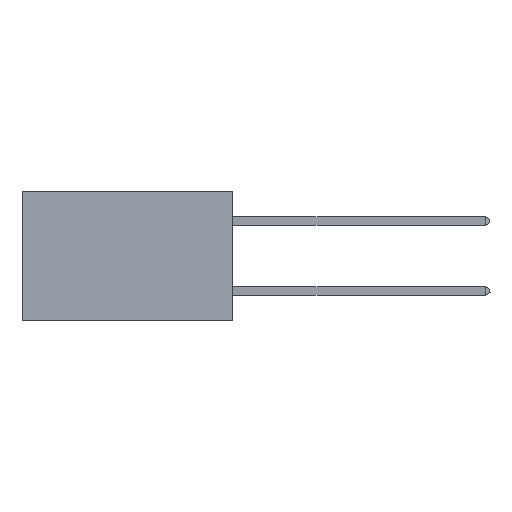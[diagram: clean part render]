
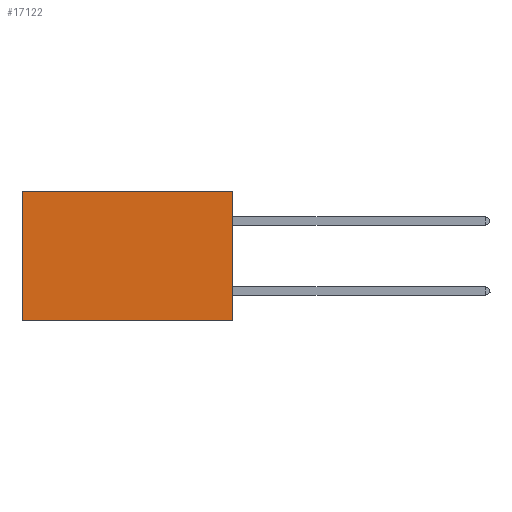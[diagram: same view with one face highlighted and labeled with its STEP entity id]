
A CAD part, left-side view. The second image highlights one B-rep face of the part: STEP entity #17122.
In plain terms, the highlighted planar face has unit normal (-1, 0, 0).
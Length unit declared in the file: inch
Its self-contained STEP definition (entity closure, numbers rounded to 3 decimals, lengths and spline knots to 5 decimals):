
#410 = CARTESIAN_POINT ( 'NONE',  ( 0.2875, 0., 0. ) ) ;
#444 = VECTOR ( 'NONE', #18063, 39.37008 ) ;
#1239 = AXIS2_PLACEMENT_3D ( 'NONE', #410, #4555, #22601 ) ;
#1261 = ORIENTED_EDGE ( 'NONE', *, *, #9656, .F. ) ;
#2017 = VERTEX_POINT ( 'NONE', #3758 ) ;
#2176 = VERTEX_POINT ( 'NONE', #23910 ) ;
#2484 = LINE ( 'NONE', #21945, #3173 ) ;
#2955 = ORIENTED_EDGE ( 'NONE', *, *, #11983, .T. ) ;
#3173 = VECTOR ( 'NONE', #3385, 39.37008 ) ;
#3385 = DIRECTION ( 'NONE',  ( 0., 0., -1. ) ) ;
#3758 = CARTESIAN_POINT ( 'NONE',  ( 0.2875, 0., -0.37 ) ) ;
#4555 = DIRECTION ( 'NONE',  ( 1., 0., 0. ) ) ;
#4723 = LINE ( 'NONE', #9162, #11554 ) ;
#4982 = FACE_OUTER_BOUND ( 'NONE', #17335, .T. ) ;
#5604 = CARTESIAN_POINT ( 'NONE',  ( 0.2875, 0.6, 0. ) ) ;
#6593 = CARTESIAN_POINT ( 'NONE',  ( 0.2875, 0., 0. ) ) ;
#6716 = CARTESIAN_POINT ( 'NONE',  ( 0.2875, 0., -0.37 ) ) ;
#8012 = EDGE_CURVE ( 'NONE', #2017, #2176, #18473, .T. ) ;
#9162 = CARTESIAN_POINT ( 'NONE',  ( 0.2875, 0., 0. ) ) ;
#9379 = VERTEX_POINT ( 'NONE', #23831 ) ;
#9656 = EDGE_CURVE ( 'NONE', #18750, #2017, #2484, .T. ) ;
#9981 = EDGE_CURVE ( 'NONE', #18750, #9379, #4723, .T. ) ;
#11554 = VECTOR ( 'NONE', #23411, 39.37008 ) ;
#11983 = EDGE_CURVE ( 'NONE', #9379, #2176, #19591, .T. ) ;
#15023 = ORIENTED_EDGE ( 'NONE', *, *, #9981, .T. ) ;
#15224 = VECTOR ( 'NONE', #25496, 39.37008 ) ;
#16563 = PLANE ( 'NONE',  #1239 ) ;
#17122 = ADVANCED_FACE ( 'NONE', ( #4982 ), #16563, .F. ) ;
#17335 = EDGE_LOOP ( 'NONE', ( #2955, #19024, #1261, #15023 ) ) ;
#18063 = DIRECTION ( 'NONE',  ( 0., 0., -1. ) ) ;
#18473 = LINE ( 'NONE', #6716, #15224 ) ;
#18750 = VERTEX_POINT ( 'NONE', #6593 ) ;
#19024 = ORIENTED_EDGE ( 'NONE', *, *, #8012, .F. ) ;
#19591 = LINE ( 'NONE', #5604, #444 ) ;
#21945 = CARTESIAN_POINT ( 'NONE',  ( 0.2875, 0., 0. ) ) ;
#22601 = DIRECTION ( 'NONE',  ( 0., 0., -1. ) ) ;
#23411 = DIRECTION ( 'NONE',  ( 0., 1., 0. ) ) ;
#23831 = CARTESIAN_POINT ( 'NONE',  ( 0.2875, 0.6, 0. ) ) ;
#23910 = CARTESIAN_POINT ( 'NONE',  ( 0.2875, 0.6, -0.37 ) ) ;
#25496 = DIRECTION ( 'NONE',  ( 0., 1., 0. ) ) ;
